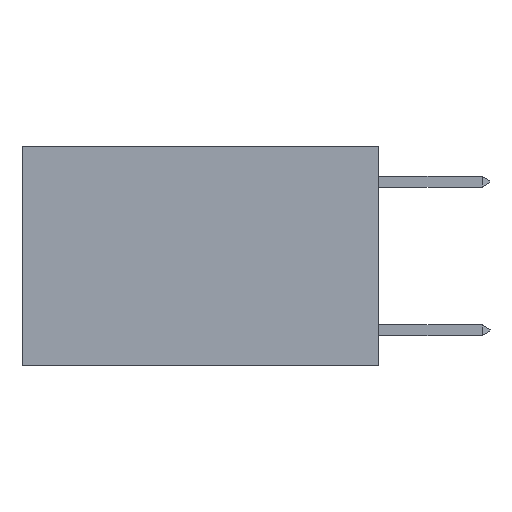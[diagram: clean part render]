
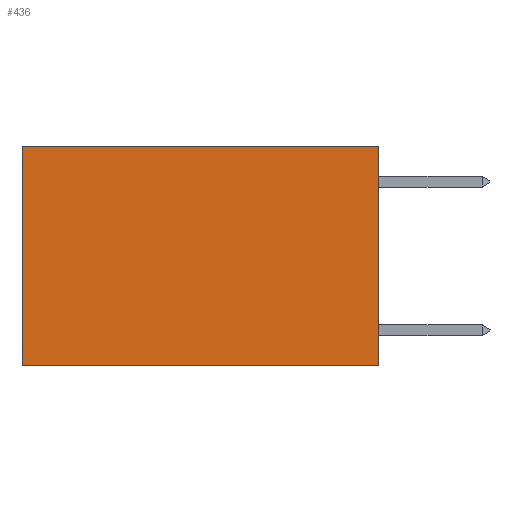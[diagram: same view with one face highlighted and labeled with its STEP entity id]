
A CAD part, left-side view. The second image highlights one B-rep face of the part: STEP entity #436.
In plain terms, the highlighted planar face has unit normal (-1, 0, 0).
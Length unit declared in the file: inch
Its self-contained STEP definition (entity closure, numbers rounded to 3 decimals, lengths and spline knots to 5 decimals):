
#436 = ADVANCED_FACE ( 'NONE', ( #3881 ), #16574, .F. ) ;
#449 = CARTESIAN_POINT ( 'NONE',  ( 0.2625, 0.6, -0.37 ) ) ;
#2390 = DIRECTION ( 'NONE',  ( 1., 0., 0. ) ) ;
#2397 = VECTOR ( 'NONE', #13214, 39.37008 ) ;
#2402 = LINE ( 'NONE', #18941, #2397 ) ;
#3517 = DIRECTION ( 'NONE',  ( 0., 1., 0. ) ) ;
#3881 = FACE_OUTER_BOUND ( 'NONE', #19706, .T. ) ;
#4534 = VERTEX_POINT ( 'NONE', #9129 ) ;
#4636 = ORIENTED_EDGE ( 'NONE', *, *, #12740, .F. ) ;
#4847 = CARTESIAN_POINT ( 'NONE',  ( 0.2625, 0., 0. ) ) ;
#5213 = EDGE_CURVE ( 'NONE', #4534, #13387, #10075, .T. ) ;
#5346 = EDGE_CURVE ( 'NONE', #16731, #14539, #6205, .T. ) ;
#6054 = VECTOR ( 'NONE', #15344, 39.37008 ) ;
#6205 = LINE ( 'NONE', #15363, #6054 ) ;
#6216 = DIRECTION ( 'NONE',  ( 0., 0., -1. ) ) ;
#6885 = CARTESIAN_POINT ( 'NONE',  ( 0.2625, 0., -0.37 ) ) ;
#9074 = ORIENTED_EDGE ( 'NONE', *, *, #19268, .T. ) ;
#9129 = CARTESIAN_POINT ( 'NONE',  ( 0.2625, 0.6, 0. ) ) ;
#9276 = VECTOR ( 'NONE', #16607, 39.37008 ) ;
#10075 = LINE ( 'NONE', #16769, #9276 ) ;
#12740 = EDGE_CURVE ( 'NONE', #14539, #13387, #19482, .T. ) ;
#13214 = DIRECTION ( 'NONE',  ( 0., 1., 0. ) ) ;
#13387 = VERTEX_POINT ( 'NONE', #449 ) ;
#14539 = VERTEX_POINT ( 'NONE', #18493 ) ;
#15199 = ORIENTED_EDGE ( 'NONE', *, *, #5346, .F. ) ;
#15344 = DIRECTION ( 'NONE',  ( 0., 0., -1. ) ) ;
#15363 = CARTESIAN_POINT ( 'NONE',  ( 0.2625, 0., 0. ) ) ;
#16574 = PLANE ( 'NONE',  #19142 ) ;
#16607 = DIRECTION ( 'NONE',  ( 0., 0., -1. ) ) ;
#16731 = VERTEX_POINT ( 'NONE', #17722 ) ;
#16769 = CARTESIAN_POINT ( 'NONE',  ( 0.2625, 0.6, 0. ) ) ;
#17722 = CARTESIAN_POINT ( 'NONE',  ( 0.2625, 0., 0. ) ) ;
#18070 = ORIENTED_EDGE ( 'NONE', *, *, #5213, .T. ) ;
#18493 = CARTESIAN_POINT ( 'NONE',  ( 0.2625, 0., -0.37 ) ) ;
#18941 = CARTESIAN_POINT ( 'NONE',  ( 0.2625, 0., 0. ) ) ;
#19142 = AXIS2_PLACEMENT_3D ( 'NONE', #4847, #2390, #6216 ) ;
#19268 = EDGE_CURVE ( 'NONE', #16731, #4534, #2402, .T. ) ;
#19482 = LINE ( 'NONE', #6885, #19585 ) ;
#19585 = VECTOR ( 'NONE', #3517, 39.37008 ) ;
#19706 = EDGE_LOOP ( 'NONE', ( #18070, #4636, #15199, #9074 ) ) ;
